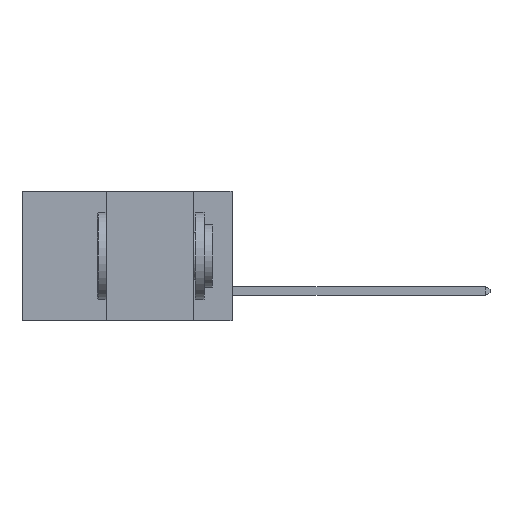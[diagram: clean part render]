
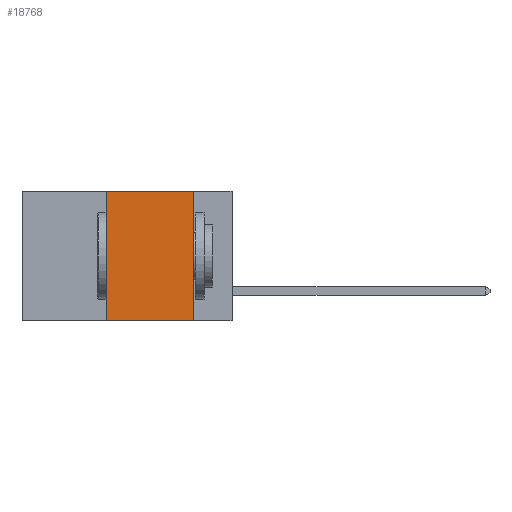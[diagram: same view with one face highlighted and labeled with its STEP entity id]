
A CAD part, left-side view. The second image highlights one B-rep face of the part: STEP entity #18768.
In plain terms, the highlighted planar face has unit normal (-1, 0, 0).
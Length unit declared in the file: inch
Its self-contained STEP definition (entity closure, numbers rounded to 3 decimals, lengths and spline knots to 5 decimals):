
#77 = VERTEX_POINT ( 'NONE', #14703 ) ;
#759 = EDGE_CURVE ( 'NONE', #12365, #6623, #14688, .T. ) ;
#982 = EDGE_CURVE ( 'NONE', #77, #10311, #3185, .T. ) ;
#2768 = EDGE_LOOP ( 'NONE', ( #9998, #12322, #18467, #16564 ) ) ;
#3185 = LINE ( 'NONE', #12196, #18147 ) ;
#3315 = PLANE ( 'NONE',  #9824 ) ;
#3680 = CARTESIAN_POINT ( 'NONE',  ( 0., 0.11, 0. ) ) ;
#5024 = VECTOR ( 'NONE', #18333, 39.37008 ) ;
#6323 = DIRECTION ( 'NONE',  ( 0., 0., -1. ) ) ;
#6623 = VERTEX_POINT ( 'NONE', #17713 ) ;
#6630 = EDGE_CURVE ( 'NONE', #77, #12365, #16160, .T. ) ;
#6944 = VECTOR ( 'NONE', #16397, 39.37008 ) ;
#9824 = AXIS2_PLACEMENT_3D ( 'NONE', #17764, #15040, #6323 ) ;
#9998 = ORIENTED_EDGE ( 'NONE', *, *, #14454, .F. ) ;
#10311 = VERTEX_POINT ( 'NONE', #11940 ) ;
#11717 = DIRECTION ( 'NONE',  ( 0., -1., 0. ) ) ;
#11940 = CARTESIAN_POINT ( 'NONE',  ( 0., 0.11, -0.37 ) ) ;
#12196 = CARTESIAN_POINT ( 'NONE',  ( 0., 0.6, -0.37 ) ) ;
#12322 = ORIENTED_EDGE ( 'NONE', *, *, #759, .F. ) ;
#12365 = VERTEX_POINT ( 'NONE', #12454 ) ;
#12454 = CARTESIAN_POINT ( 'NONE',  ( 0., 0.36, 0. ) ) ;
#12906 = LINE ( 'NONE', #3680, #13808 ) ;
#13646 = FACE_OUTER_BOUND ( 'NONE', #2768, .T. ) ;
#13808 = VECTOR ( 'NONE', #15322, 39.37008 ) ;
#14454 = EDGE_CURVE ( 'NONE', #6623, #10311, #12906, .T. ) ;
#14688 = LINE ( 'NONE', #16541, #6944 ) ;
#14703 = CARTESIAN_POINT ( 'NONE',  ( 0., 0.36, -0.37 ) ) ;
#15040 = DIRECTION ( 'NONE',  ( 1., 0., 0. ) ) ;
#15322 = DIRECTION ( 'NONE',  ( 0., 0., -1. ) ) ;
#16160 = LINE ( 'NONE', #17446, #5024 ) ;
#16397 = DIRECTION ( 'NONE',  ( 0., -1., 0. ) ) ;
#16541 = CARTESIAN_POINT ( 'NONE',  ( 0., 0.6, 0. ) ) ;
#16564 = ORIENTED_EDGE ( 'NONE', *, *, #982, .T. ) ;
#17446 = CARTESIAN_POINT ( 'NONE',  ( 0., 0.36, 0. ) ) ;
#17713 = CARTESIAN_POINT ( 'NONE',  ( 0., 0.11, 0. ) ) ;
#17764 = CARTESIAN_POINT ( 'NONE',  ( 0., 0.6, 0. ) ) ;
#18147 = VECTOR ( 'NONE', #11717, 39.37008 ) ;
#18333 = DIRECTION ( 'NONE',  ( 0., 0., 1. ) ) ;
#18467 = ORIENTED_EDGE ( 'NONE', *, *, #6630, .F. ) ;
#18768 = ADVANCED_FACE ( 'NONE', ( #13646 ), #3315, .F. ) ;
